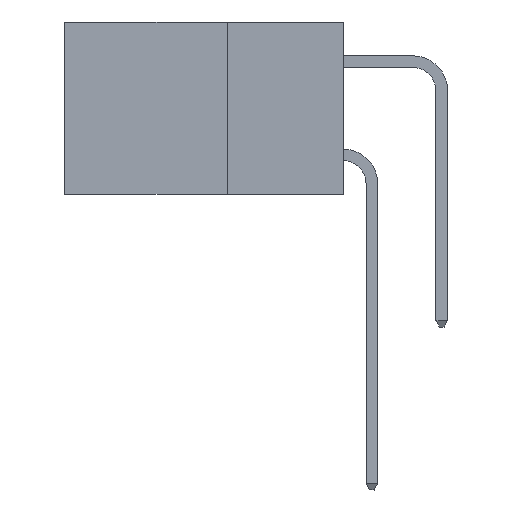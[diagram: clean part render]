
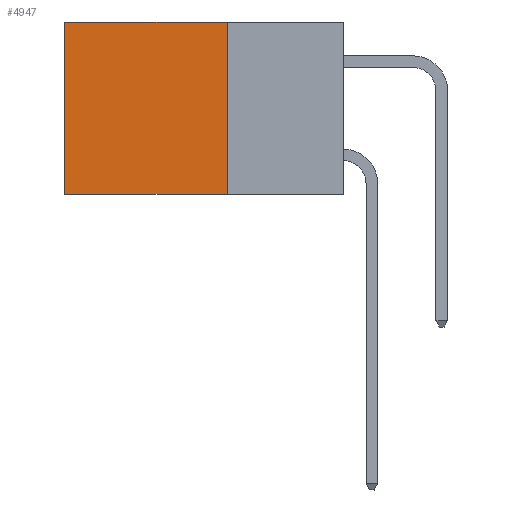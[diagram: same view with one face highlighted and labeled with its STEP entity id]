
A CAD part, left-side view. The second image highlights one B-rep face of the part: STEP entity #4947.
In plain terms, the highlighted planar face has unit normal (-1, 0, 0).
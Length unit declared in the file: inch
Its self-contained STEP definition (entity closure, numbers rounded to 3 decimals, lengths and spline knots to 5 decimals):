
#581 = CARTESIAN_POINT ( 'NONE',  ( 0.2615, 0.6, -0.37 ) ) ;
#805 = EDGE_CURVE ( 'NONE', #2232, #13869, #10154, .T. ) ;
#821 = CARTESIAN_POINT ( 'NONE',  ( 0.2615, 0.25, 0. ) ) ;
#1028 = DIRECTION ( 'NONE',  ( 0., 0., -1. ) ) ;
#1218 = ORIENTED_EDGE ( 'NONE', *, *, #14654, .F. ) ;
#2136 = CARTESIAN_POINT ( 'NONE',  ( 0.2615, 0.6, -0.37 ) ) ;
#2179 = VECTOR ( 'NONE', #2424, 39.37008 ) ;
#2232 = VERTEX_POINT ( 'NONE', #13697 ) ;
#2424 = DIRECTION ( 'NONE',  ( 0., 1., 0. ) ) ;
#3230 = VERTEX_POINT ( 'NONE', #10190 ) ;
#3673 = CARTESIAN_POINT ( 'NONE',  ( 0.2615, 0.25, -0.37 ) ) ;
#4040 = PLANE ( 'NONE',  #14335 ) ;
#4109 = LINE ( 'NONE', #7978, #6139 ) ;
#4613 = LINE ( 'NONE', #821, #5703 ) ;
#4728 = LINE ( 'NONE', #2136, #8648 ) ;
#4947 = ADVANCED_FACE ( 'NONE', ( #6582 ), #4040, .F. ) ;
#5703 = VECTOR ( 'NONE', #10834, 39.37008 ) ;
#5896 = EDGE_CURVE ( 'NONE', #3230, #6083, #4613, .T. ) ;
#6083 = VERTEX_POINT ( 'NONE', #16053 ) ;
#6084 = EDGE_CURVE ( 'NONE', #6083, #13869, #4728, .T. ) ;
#6139 = VECTOR ( 'NONE', #6891, 39.37008 ) ;
#6538 = ORIENTED_EDGE ( 'NONE', *, *, #5896, .T. ) ;
#6582 = FACE_OUTER_BOUND ( 'NONE', #7507, .T. ) ;
#6891 = DIRECTION ( 'NONE',  ( 0., 0., -1. ) ) ;
#7507 = EDGE_LOOP ( 'NONE', ( #8681, #13764, #1218, #6538 ) ) ;
#7978 = CARTESIAN_POINT ( 'NONE',  ( 0.2615, 0.25, -0.37 ) ) ;
#8648 = VECTOR ( 'NONE', #1028, 39.37008 ) ;
#8681 = ORIENTED_EDGE ( 'NONE', *, *, #6084, .T. ) ;
#9167 = CARTESIAN_POINT ( 'NONE',  ( 0.2615, 0.25, -0.37 ) ) ;
#10154 = LINE ( 'NONE', #3673, #2179 ) ;
#10190 = CARTESIAN_POINT ( 'NONE',  ( 0.2615, 0.25, 0. ) ) ;
#10834 = DIRECTION ( 'NONE',  ( 0., 1., 0. ) ) ;
#13697 = CARTESIAN_POINT ( 'NONE',  ( 0.2615, 0.25, -0.37 ) ) ;
#13764 = ORIENTED_EDGE ( 'NONE', *, *, #805, .F. ) ;
#13869 = VERTEX_POINT ( 'NONE', #581 ) ;
#14311 = DIRECTION ( 'NONE',  ( 1., 0., 0. ) ) ;
#14335 = AXIS2_PLACEMENT_3D ( 'NONE', #9167, #14311, #15689 ) ;
#14654 = EDGE_CURVE ( 'NONE', #3230, #2232, #4109, .T. ) ;
#15689 = DIRECTION ( 'NONE',  ( 0., 0., -1. ) ) ;
#16053 = CARTESIAN_POINT ( 'NONE',  ( 0.2615, 0.6, 0. ) ) ;
